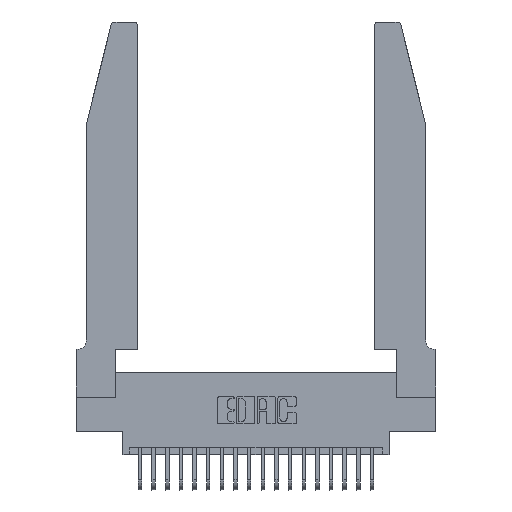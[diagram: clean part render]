
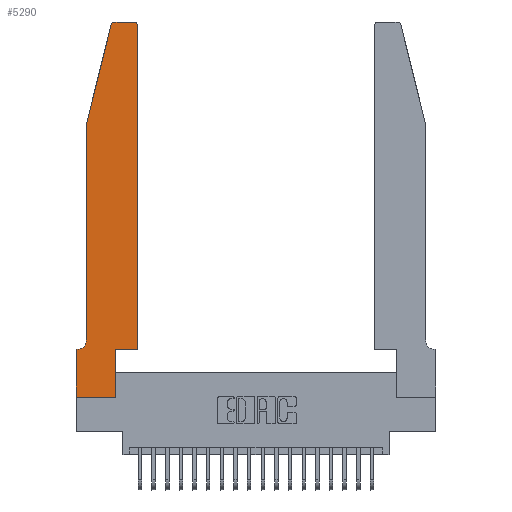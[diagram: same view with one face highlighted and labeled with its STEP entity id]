
A CAD part, top view. The second image highlights one B-rep face of the part: STEP entity #5290.
In plain terms, the highlighted planar face has unit normal (0, 0, 1).
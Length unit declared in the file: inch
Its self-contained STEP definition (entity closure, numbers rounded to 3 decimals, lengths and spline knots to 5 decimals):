
#41 = PLANE ( 'NONE',  #4613 ) ;
#606 = ORIENTED_EDGE ( 'NONE', *, *, #3268, .T. ) ;
#635 = EDGE_CURVE ( 'NONE', #7911, #13416, #3851, .T. ) ;
#659 = DIRECTION ( 'NONE',  ( -1., 0., 0. ) ) ;
#1445 = DIRECTION ( 'NONE',  ( -0.239, -0.971, 0. ) ) ;
#1500 = LINE ( 'NONE', #19852, #14465 ) ;
#1796 = DIRECTION ( 'NONE',  ( 1., 0., 0. ) ) ;
#1998 = VERTEX_POINT ( 'NONE', #7894 ) ;
#2519 = AXIS2_PLACEMENT_3D ( 'NONE', #9908, #21479, #11613 ) ;
#3100 = CARTESIAN_POINT ( 'NONE',  ( 0.0755, 0.42, 0.37 ) ) ;
#3267 = LINE ( 'NONE', #9507, #16177 ) ;
#3268 = EDGE_CURVE ( 'NONE', #12309, #6673, #3774, .T. ) ;
#3374 = VERTEX_POINT ( 'NONE', #6423 ) ;
#3774 = LINE ( 'NONE', #14484, #15613 ) ;
#3851 = LINE ( 'NONE', #14158, #16727 ) ;
#3879 = CARTESIAN_POINT ( 'NONE',  ( 0., 0., 0.37 ) ) ;
#4465 = EDGE_CURVE ( 'NONE', #14769, #12309, #1500, .T. ) ;
#4513 = DIRECTION ( 'NONE',  ( 0., 1., 0. ) ) ;
#4613 = AXIS2_PLACEMENT_3D ( 'NONE', #5208, #11989, #1796 ) ;
#5203 = CARTESIAN_POINT ( 'NONE',  ( 0.2865, 0., 0.37 ) ) ;
#5208 = CARTESIAN_POINT ( 'NONE',  ( 0., 0.35, 0.37 ) ) ;
#5290 = ADVANCED_FACE ( 'NONE', ( #14471 ), #41, .T. ) ;
#5891 = EDGE_CURVE ( 'NONE', #12208, #7681, #15754, .T. ) ;
#6240 = CARTESIAN_POINT ( 'NONE',  ( 0., 0.35, 0.37 ) ) ;
#6296 = ORIENTED_EDGE ( 'NONE', *, *, #7672, .T. ) ;
#6416 = VERTEX_POINT ( 'NONE', #3100 ) ;
#6423 = CARTESIAN_POINT ( 'NONE',  ( 0.4505, 2.72, 0.37 ) ) ;
#6620 = DIRECTION ( 'NONE',  ( 1., 0., 0. ) ) ;
#6673 = VERTEX_POINT ( 'NONE', #16726 ) ;
#6677 = VECTOR ( 'NONE', #9277, 39.37008 ) ;
#6796 = DIRECTION ( 'NONE',  ( 0., 0., -1. ) ) ;
#6854 = VECTOR ( 'NONE', #13681, 39.37008 ) ;
#7227 = CARTESIAN_POINT ( 'NONE',  ( 0.25487, 2.72718, 0.37 ) ) ;
#7282 = ORIENTED_EDGE ( 'NONE', *, *, #13261, .T. ) ;
#7585 = CARTESIAN_POINT ( 'NONE',  ( 0.4505, 0.35, 0.37 ) ) ;
#7672 = EDGE_CURVE ( 'NONE', #6673, #16412, #12819, .T. ) ;
#7681 = VERTEX_POINT ( 'NONE', #18024 ) ;
#7894 = CARTESIAN_POINT ( 'NONE',  ( 0.0755, 2., 0.37 ) ) ;
#7911 = VERTEX_POINT ( 'NONE', #10343 ) ;
#8220 = ORIENTED_EDGE ( 'NONE', *, *, #15431, .T. ) ;
#8256 = EDGE_CURVE ( 'NONE', #13416, #14769, #3267, .T. ) ;
#8625 = CARTESIAN_POINT ( 'NONE',  ( 0.2605, 2.75, 0.37 ) ) ;
#8750 = LINE ( 'NONE', #13972, #17098 ) ;
#8981 = LINE ( 'NONE', #19928, #21685 ) ;
#9028 = EDGE_LOOP ( 'NONE', ( #11065, #19309, #8220, #11450, #9492, #19997, #18147, #19492, #606, #6296, #7282, #14270 ) ) ;
#9033 = CARTESIAN_POINT ( 'NONE',  ( 0.284, 2.72, 0.37 ) ) ;
#9210 = AXIS2_PLACEMENT_3D ( 'NONE', #16817, #6796, #18427 ) ;
#9277 = DIRECTION ( 'NONE',  ( 0., 1., 0. ) ) ;
#9492 = ORIENTED_EDGE ( 'NONE', *, *, #17664, .T. ) ;
#9507 = CARTESIAN_POINT ( 'NONE',  ( 0., 0., 0.37 ) ) ;
#9519 = CARTESIAN_POINT ( 'NONE',  ( 0.4505, 0.35, 0.37 ) ) ;
#9908 = CARTESIAN_POINT ( 'NONE',  ( 0.4205, 2.72, 0.37 ) ) ;
#10343 = CARTESIAN_POINT ( 'NONE',  ( 0.0055, 0.35, 0.37 ) ) ;
#10720 = DIRECTION ( 'NONE',  ( 1., 0., 0. ) ) ;
#10919 = AXIS2_PLACEMENT_3D ( 'NONE', #9033, #20621, #10720 ) ;
#11065 = ORIENTED_EDGE ( 'NONE', *, *, #5891, .T. ) ;
#11384 = CARTESIAN_POINT ( 'NONE',  ( 0.4505, 0.35, 0.37 ) ) ;
#11450 = ORIENTED_EDGE ( 'NONE', *, *, #14748, .T. ) ;
#11613 = DIRECTION ( 'NONE',  ( 1., 0., 0. ) ) ;
#11704 = LINE ( 'NONE', #7585, #6677 ) ;
#11989 = DIRECTION ( 'NONE',  ( 0., 0., 1. ) ) ;
#12167 = EDGE_CURVE ( 'NONE', #3374, #12208, #20762, .T. ) ;
#12208 = VERTEX_POINT ( 'NONE', #13345 ) ;
#12309 = VERTEX_POINT ( 'NONE', #5203 ) ;
#12819 = LINE ( 'NONE', #11384, #17221 ) ;
#13261 = EDGE_CURVE ( 'NONE', #16412, #3374, #11704, .T. ) ;
#13345 = CARTESIAN_POINT ( 'NONE',  ( 0.4205, 2.75, 0.37 ) ) ;
#13416 = VERTEX_POINT ( 'NONE', #6240 ) ;
#13681 = DIRECTION ( 'NONE',  ( -1., 0., 0. ) ) ;
#13972 = CARTESIAN_POINT ( 'NONE',  ( 0.0755, 2., 0.37 ) ) ;
#14158 = CARTESIAN_POINT ( 'NONE',  ( 0.0755, 0.35, 0.37 ) ) ;
#14270 = ORIENTED_EDGE ( 'NONE', *, *, #12167, .T. ) ;
#14465 = VECTOR ( 'NONE', #6620, 39.37008 ) ;
#14471 = FACE_OUTER_BOUND ( 'NONE', #9028, .T. ) ;
#14484 = CARTESIAN_POINT ( 'NONE',  ( 0.2865, 0.35, 0.37 ) ) ;
#14544 = DIRECTION ( 'NONE',  ( 0., -1., 0. ) ) ;
#14748 = EDGE_CURVE ( 'NONE', #1998, #6416, #8750, .T. ) ;
#14769 = VERTEX_POINT ( 'NONE', #3879 ) ;
#15222 = CIRCLE ( 'NONE', #9210, 0.07 ) ;
#15431 = EDGE_CURVE ( 'NONE', #17842, #1998, #8981, .T. ) ;
#15613 = VECTOR ( 'NONE', #4513, 39.37008 ) ;
#15645 = DIRECTION ( 'NONE',  ( 0., -1., 0. ) ) ;
#15754 = LINE ( 'NONE', #8625, #6854 ) ;
#16177 = VECTOR ( 'NONE', #14544, 39.37008 ) ;
#16412 = VERTEX_POINT ( 'NONE', #9519 ) ;
#16726 = CARTESIAN_POINT ( 'NONE',  ( 0.2865, 0.35, 0.37 ) ) ;
#16727 = VECTOR ( 'NONE', #659, 39.37008 ) ;
#16817 = CARTESIAN_POINT ( 'NONE',  ( 0.0055, 0.42, 0.37 ) ) ;
#17098 = VECTOR ( 'NONE', #15645, 39.37008 ) ;
#17221 = VECTOR ( 'NONE', #21260, 39.37008 ) ;
#17664 = EDGE_CURVE ( 'NONE', #6416, #7911, #15222, .T. ) ;
#17842 = VERTEX_POINT ( 'NONE', #7227 ) ;
#18024 = CARTESIAN_POINT ( 'NONE',  ( 0.284, 2.75, 0.37 ) ) ;
#18147 = ORIENTED_EDGE ( 'NONE', *, *, #8256, .T. ) ;
#18427 = DIRECTION ( 'NONE',  ( -1., 0., 0. ) ) ;
#19080 = EDGE_CURVE ( 'NONE', #7681, #17842, #21306, .T. ) ;
#19309 = ORIENTED_EDGE ( 'NONE', *, *, #19080, .T. ) ;
#19492 = ORIENTED_EDGE ( 'NONE', *, *, #4465, .T. ) ;
#19852 = CARTESIAN_POINT ( 'NONE',  ( 0., 0., 0.37 ) ) ;
#19928 = CARTESIAN_POINT ( 'NONE',  ( 0.0755, 2., 0.37 ) ) ;
#19997 = ORIENTED_EDGE ( 'NONE', *, *, #635, .T. ) ;
#20621 = DIRECTION ( 'NONE',  ( 0., 0., 1. ) ) ;
#20762 = CIRCLE ( 'NONE', #2519, 0.03 ) ;
#21260 = DIRECTION ( 'NONE',  ( 1., 0., 0. ) ) ;
#21306 = CIRCLE ( 'NONE', #10919, 0.03 ) ;
#21479 = DIRECTION ( 'NONE',  ( 0., 0., 1. ) ) ;
#21685 = VECTOR ( 'NONE', #1445, 39.37008 ) ;
